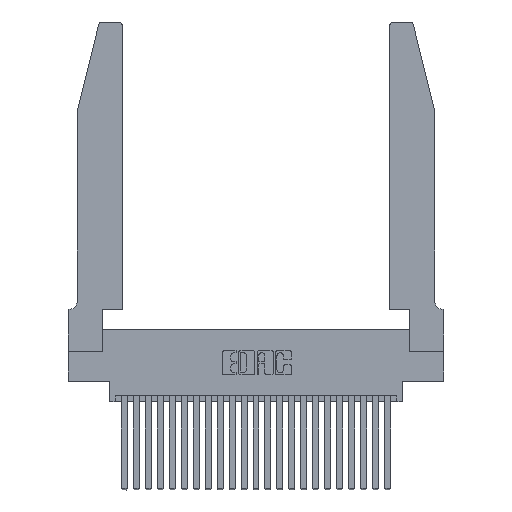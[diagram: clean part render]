
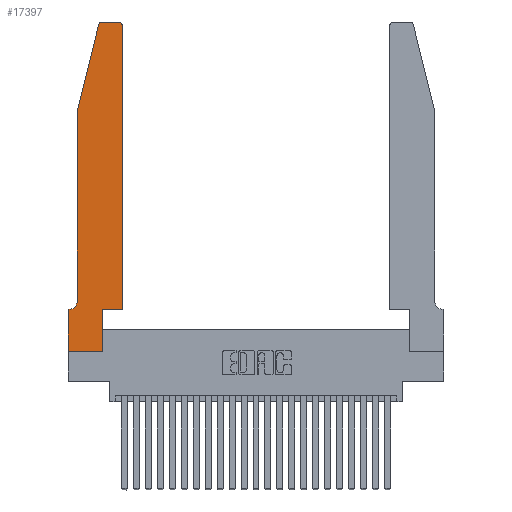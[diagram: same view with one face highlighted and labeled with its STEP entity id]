
A CAD part, top view. The second image highlights one B-rep face of the part: STEP entity #17397.
In plain terms, the highlighted planar face has unit normal (0, 0, 1).
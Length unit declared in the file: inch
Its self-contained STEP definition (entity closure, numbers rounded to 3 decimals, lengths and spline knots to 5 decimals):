
#174 = VERTEX_POINT ( 'NONE', #13723 ) ;
#380 = ORIENTED_EDGE ( 'NONE', *, *, #23236, .T. ) ;
#634 = EDGE_CURVE ( 'NONE', #20629, #11599, #11152, .T. ) ;
#1325 = CARTESIAN_POINT ( 'NONE',  ( 0., 0., 0.37 ) ) ;
#1644 = CARTESIAN_POINT ( 'NONE',  ( 0.4505, 0.35, 0.37 ) ) ;
#1707 = DIRECTION ( 'NONE',  ( 0., 0., -1. ) ) ;
#1873 = LINE ( 'NONE', #1995, #13772 ) ;
#1945 = VECTOR ( 'NONE', #3396, 39.37008 ) ;
#1995 = CARTESIAN_POINT ( 'NONE',  ( 0.2865, 0.35, 0.37 ) ) ;
#2243 = VERTEX_POINT ( 'NONE', #25273 ) ;
#2669 = DIRECTION ( 'NONE',  ( 0., 0., 1. ) ) ;
#3219 = VERTEX_POINT ( 'NONE', #8234 ) ;
#3396 = DIRECTION ( 'NONE',  ( -1., 0., 0. ) ) ;
#3511 = CARTESIAN_POINT ( 'NONE',  ( 0., 0., 0.37 ) ) ;
#3579 = EDGE_CURVE ( 'NONE', #174, #10648, #19549, .T. ) ;
#3696 = EDGE_CURVE ( 'NONE', #11599, #7338, #11035, .T. ) ;
#3868 = VERTEX_POINT ( 'NONE', #8364 ) ;
#3940 = ORIENTED_EDGE ( 'NONE', *, *, #21512, .T. ) ;
#3997 = DIRECTION ( 'NONE',  ( 0., 1., 0. ) ) ;
#4014 = ORIENTED_EDGE ( 'NONE', *, *, #21270, .T. ) ;
#4273 = FACE_OUTER_BOUND ( 'NONE', #17993, .T. ) ;
#5129 = CARTESIAN_POINT ( 'NONE',  ( 0.0755, 2., 0.37 ) ) ;
#5227 = CARTESIAN_POINT ( 'NONE',  ( 0., 0.35, 0.37 ) ) ;
#6172 = ORIENTED_EDGE ( 'NONE', *, *, #11651, .T. ) ;
#6315 = CARTESIAN_POINT ( 'NONE',  ( 0.284, 2.75, 0.37 ) ) ;
#6609 = EDGE_CURVE ( 'NONE', #7338, #174, #14676, .T. ) ;
#6745 = AXIS2_PLACEMENT_3D ( 'NONE', #17144, #13536, #7710 ) ;
#6764 = LINE ( 'NONE', #1325, #14979 ) ;
#6806 = EDGE_CURVE ( 'NONE', #11073, #13822, #13718, .T. ) ;
#6900 = CARTESIAN_POINT ( 'NONE',  ( 0., 0., 0.37 ) ) ;
#6963 = PLANE ( 'NONE',  #20251 ) ;
#7338 = VERTEX_POINT ( 'NONE', #13216 ) ;
#7382 = DIRECTION ( 'NONE',  ( 1., 0., 0. ) ) ;
#7663 = CIRCLE ( 'NONE', #22899, 0.07 ) ;
#7710 = DIRECTION ( 'NONE',  ( 1., 0., 0. ) ) ;
#7824 = ORIENTED_EDGE ( 'NONE', *, *, #6806, .T. ) ;
#8048 = DIRECTION ( 'NONE',  ( -1., 0., 0. ) ) ;
#8073 = CIRCLE ( 'NONE', #6745, 0.03 ) ;
#8234 = CARTESIAN_POINT ( 'NONE',  ( 0.0055, 0.35, 0.37 ) ) ;
#8364 = CARTESIAN_POINT ( 'NONE',  ( 0.2865, 0., 0.37 ) ) ;
#8429 = CARTESIAN_POINT ( 'NONE',  ( 0.4505, 0.35, 0.37 ) ) ;
#8456 = ORIENTED_EDGE ( 'NONE', *, *, #22652, .T. ) ;
#9203 = CARTESIAN_POINT ( 'NONE',  ( 0.4205, 2.75, 0.37 ) ) ;
#9397 = DIRECTION ( 'NONE',  ( 0., -1., 0. ) ) ;
#9940 = VECTOR ( 'NONE', #15396, 39.37008 ) ;
#10648 = VERTEX_POINT ( 'NONE', #20238 ) ;
#10721 = DIRECTION ( 'NONE',  ( 1., 0., 0. ) ) ;
#11035 = CIRCLE ( 'NONE', #16603, 0.03 ) ;
#11073 = VERTEX_POINT ( 'NONE', #19102 ) ;
#11152 = LINE ( 'NONE', #15072, #1945 ) ;
#11545 = LINE ( 'NONE', #14027, #16089 ) ;
#11599 = VERTEX_POINT ( 'NONE', #6315 ) ;
#11651 = EDGE_CURVE ( 'NONE', #3219, #22309, #11545, .T. ) ;
#12222 = ORIENTED_EDGE ( 'NONE', *, *, #3696, .T. ) ;
#12373 = DIRECTION ( 'NONE',  ( 0., 1., 0. ) ) ;
#12402 = CARTESIAN_POINT ( 'NONE',  ( 0., 0.35, 0.37 ) ) ;
#13144 = VECTOR ( 'NONE', #24777, 39.37008 ) ;
#13216 = CARTESIAN_POINT ( 'NONE',  ( 0.25487, 2.72718, 0.37 ) ) ;
#13536 = DIRECTION ( 'NONE',  ( 0., 0., 1. ) ) ;
#13573 = EDGE_CURVE ( 'NONE', #2243, #11073, #17849, .T. ) ;
#13718 = LINE ( 'NONE', #8429, #20171 ) ;
#13723 = CARTESIAN_POINT ( 'NONE',  ( 0.0755, 2., 0.37 ) ) ;
#13772 = VECTOR ( 'NONE', #3997, 39.37008 ) ;
#13822 = VERTEX_POINT ( 'NONE', #18503 ) ;
#13851 = ORIENTED_EDGE ( 'NONE', *, *, #21233, .T. ) ;
#14027 = CARTESIAN_POINT ( 'NONE',  ( 0.0755, 0.35, 0.37 ) ) ;
#14676 = LINE ( 'NONE', #5129, #13144 ) ;
#14809 = ORIENTED_EDGE ( 'NONE', *, *, #13573, .T. ) ;
#14979 = VECTOR ( 'NONE', #20883, 39.37008 ) ;
#15072 = CARTESIAN_POINT ( 'NONE',  ( 0.2605, 2.75, 0.37 ) ) ;
#15396 = DIRECTION ( 'NONE',  ( 1., 0., 0. ) ) ;
#16089 = VECTOR ( 'NONE', #8048, 39.37008 ) ;
#16475 = ORIENTED_EDGE ( 'NONE', *, *, #6609, .T. ) ;
#16603 = AXIS2_PLACEMENT_3D ( 'NONE', #22182, #2669, #10721 ) ;
#17144 = CARTESIAN_POINT ( 'NONE',  ( 0.4205, 2.72, 0.37 ) ) ;
#17178 = DIRECTION ( 'NONE',  ( -1., 0., 0. ) ) ;
#17397 = ADVANCED_FACE ( 'NONE', ( #4273 ), #6963, .T. ) ;
#17849 = LINE ( 'NONE', #1644, #9940 ) ;
#17993 = EDGE_LOOP ( 'NONE', ( #25150, #12222, #16475, #21436, #380, #6172, #8456, #13851, #3940, #14809, #7824, #4014 ) ) ;
#18407 = VECTOR ( 'NONE', #7382, 39.37008 ) ;
#18503 = CARTESIAN_POINT ( 'NONE',  ( 0.4505, 2.72, 0.37 ) ) ;
#18651 = CARTESIAN_POINT ( 'NONE',  ( 0.0055, 0.42, 0.37 ) ) ;
#18716 = DIRECTION ( 'NONE',  ( 0., 0., 1. ) ) ;
#19102 = CARTESIAN_POINT ( 'NONE',  ( 0.4505, 0.35, 0.37 ) ) ;
#19173 = CARTESIAN_POINT ( 'NONE',  ( 0.0755, 2., 0.37 ) ) ;
#19549 = LINE ( 'NONE', #19173, #21080 ) ;
#20171 = VECTOR ( 'NONE', #12373, 39.37008 ) ;
#20238 = CARTESIAN_POINT ( 'NONE',  ( 0.0755, 0.42, 0.37 ) ) ;
#20251 = AXIS2_PLACEMENT_3D ( 'NONE', #5227, #18716, #24535 ) ;
#20545 = LINE ( 'NONE', #3511, #18407 ) ;
#20629 = VERTEX_POINT ( 'NONE', #9203 ) ;
#20883 = DIRECTION ( 'NONE',  ( 0., -1., 0. ) ) ;
#21080 = VECTOR ( 'NONE', #9397, 39.37008 ) ;
#21233 = EDGE_CURVE ( 'NONE', #24944, #3868, #20545, .T. ) ;
#21270 = EDGE_CURVE ( 'NONE', #13822, #20629, #8073, .T. ) ;
#21436 = ORIENTED_EDGE ( 'NONE', *, *, #3579, .T. ) ;
#21512 = EDGE_CURVE ( 'NONE', #3868, #2243, #1873, .T. ) ;
#22182 = CARTESIAN_POINT ( 'NONE',  ( 0.284, 2.72, 0.37 ) ) ;
#22309 = VERTEX_POINT ( 'NONE', #12402 ) ;
#22652 = EDGE_CURVE ( 'NONE', #22309, #24944, #6764, .T. ) ;
#22899 = AXIS2_PLACEMENT_3D ( 'NONE', #18651, #1707, #17178 ) ;
#23236 = EDGE_CURVE ( 'NONE', #10648, #3219, #7663, .T. ) ;
#24535 = DIRECTION ( 'NONE',  ( 1., 0., 0. ) ) ;
#24777 = DIRECTION ( 'NONE',  ( -0.239, -0.971, 0. ) ) ;
#24944 = VERTEX_POINT ( 'NONE', #6900 ) ;
#25150 = ORIENTED_EDGE ( 'NONE', *, *, #634, .T. ) ;
#25273 = CARTESIAN_POINT ( 'NONE',  ( 0.2865, 0.35, 0.37 ) ) ;
